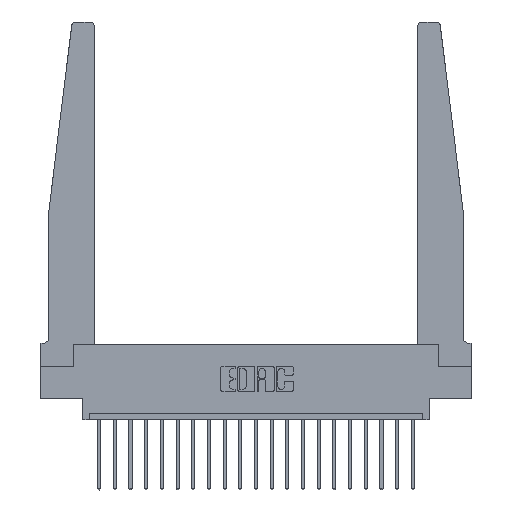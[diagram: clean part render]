
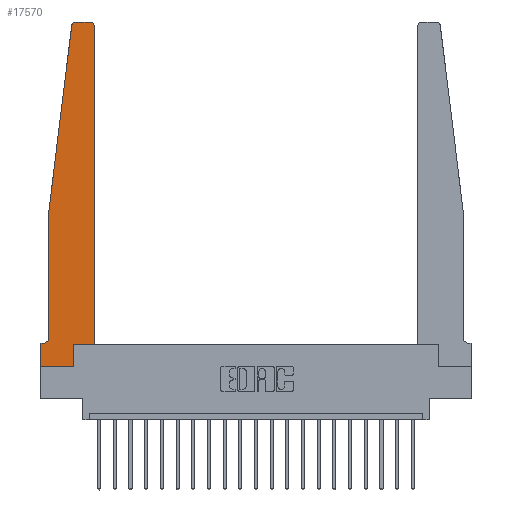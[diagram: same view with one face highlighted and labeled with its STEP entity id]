
A CAD part, top view. The second image highlights one B-rep face of the part: STEP entity #17570.
In plain terms, the highlighted planar face has unit normal (0, 0, 1).
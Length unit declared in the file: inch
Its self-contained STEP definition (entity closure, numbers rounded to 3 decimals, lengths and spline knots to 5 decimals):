
#269 = CARTESIAN_POINT ( 'NONE',  ( 0.395, 2.72, 0.37 ) ) ;
#278 = DIRECTION ( 'NONE',  ( 1., 0., 0. ) ) ;
#320 = LINE ( 'NONE', #11941, #8382 ) ;
#343 = ORIENTED_EDGE ( 'NONE', *, *, #20203, .T. ) ;
#544 = DIRECTION ( 'NONE',  ( 1., 0., 0. ) ) ;
#1042 = VERTEX_POINT ( 'NONE', #15136 ) ;
#1136 = VECTOR ( 'NONE', #544, 39.37008 ) ;
#1371 = VERTEX_POINT ( 'NONE', #17434 ) ;
#1635 = ORIENTED_EDGE ( 'NONE', *, *, #14695, .T. ) ;
#1880 = ORIENTED_EDGE ( 'NONE', *, *, #18486, .T. ) ;
#2098 = CARTESIAN_POINT ( 'NONE',  ( 0.2605, 0.18, 0.37 ) ) ;
#2448 = CARTESIAN_POINT ( 'NONE',  ( 0.015, 0.1875, 0.37 ) ) ;
#2742 = VECTOR ( 'NONE', #6853, 39.37008 ) ;
#2832 = DIRECTION ( 'NONE',  ( 0., -1., 0. ) ) ;
#3207 = EDGE_CURVE ( 'NONE', #11237, #1042, #18487, .T. ) ;
#3303 = DIRECTION ( 'NONE',  ( 0., 1., 0. ) ) ;
#3375 = CARTESIAN_POINT ( 'NONE',  ( 0.065, 1.25, 0.37 ) ) ;
#3447 = VECTOR ( 'NONE', #17825, 39.37008 ) ;
#3812 = ORIENTED_EDGE ( 'NONE', *, *, #11074, .T. ) ;
#3903 = DIRECTION ( 'NONE',  ( 1., 0., 0. ) ) ;
#4135 = EDGE_CURVE ( 'NONE', #15339, #16574, #13714, .T. ) ;
#4387 = VECTOR ( 'NONE', #2832, 39.37008 ) ;
#4436 = CARTESIAN_POINT ( 'NONE',  ( 0.015, 0.2375, 0.37 ) ) ;
#4474 = CARTESIAN_POINT ( 'NONE',  ( 0.27653, 2.75, 0.37 ) ) ;
#4518 = EDGE_CURVE ( 'NONE', #4698, #8866, #16947, .T. ) ;
#4573 = DIRECTION ( 'NONE',  ( -1., 0., 0. ) ) ;
#4656 = VECTOR ( 'NONE', #12025, 39.37008 ) ;
#4698 = VERTEX_POINT ( 'NONE', #2098 ) ;
#4708 = AXIS2_PLACEMENT_3D ( 'NONE', #16289, #14747, #278 ) ;
#4717 = DIRECTION ( 'NONE',  ( 0., 0., -1. ) ) ;
#4794 = DIRECTION ( 'NONE',  ( 0., 0., 1. ) ) ;
#4830 = CIRCLE ( 'NONE', #19026, 0.03 ) ;
#5326 = ORIENTED_EDGE ( 'NONE', *, *, #11999, .T. ) ;
#5350 = CARTESIAN_POINT ( 'NONE',  ( 0.425, 0.18, 0.37 ) ) ;
#6739 = ORIENTED_EDGE ( 'NONE', *, *, #17157, .T. ) ;
#6757 = CIRCLE ( 'NONE', #13583, 0.03 ) ;
#6811 = CARTESIAN_POINT ( 'NONE',  ( 0.27653, 2.72, 0.37 ) ) ;
#6853 = DIRECTION ( 'NONE',  ( -0.122, -0.992, 0. ) ) ;
#7519 = CARTESIAN_POINT ( 'NONE',  ( 0., 0.1875, 0.37 ) ) ;
#7604 = CARTESIAN_POINT ( 'NONE',  ( 0.065, 1.25, 0.37 ) ) ;
#7938 = EDGE_LOOP ( 'NONE', ( #10064, #1635, #12003, #343, #18929, #3812, #11332, #6739, #5326, #16904, #19817, #1880 ) ) ;
#7961 = VECTOR ( 'NONE', #3303, 39.37008 ) ;
#8055 = CARTESIAN_POINT ( 'NONE',  ( 0.24675, 2.72367, 0.37 ) ) ;
#8382 = VECTOR ( 'NONE', #15225, 39.37008 ) ;
#8735 = CARTESIAN_POINT ( 'NONE',  ( 0.25, 2.75, 0.37 ) ) ;
#8866 = VERTEX_POINT ( 'NONE', #13699 ) ;
#8931 = LINE ( 'NONE', #8735, #4656 ) ;
#9279 = EDGE_CURVE ( 'NONE', #8866, #1371, #11989, .T. ) ;
#9654 = LINE ( 'NONE', #10292, #11390 ) ;
#10027 = CARTESIAN_POINT ( 'NONE',  ( 0.065, 0.2375, 0.37 ) ) ;
#10064 = ORIENTED_EDGE ( 'NONE', *, *, #10383, .T. ) ;
#10292 = CARTESIAN_POINT ( 'NONE',  ( 0.2605, 0.18, 0.37 ) ) ;
#10306 = VECTOR ( 'NONE', #3903, 39.37008 ) ;
#10383 = EDGE_CURVE ( 'NONE', #11871, #17810, #8931, .T. ) ;
#10805 = VERTEX_POINT ( 'NONE', #3375 ) ;
#10965 = CARTESIAN_POINT ( 'NONE',  ( 0.2605, 0., 0.37 ) ) ;
#11074 = EDGE_CURVE ( 'NONE', #16574, #11237, #320, .T. ) ;
#11237 = VERTEX_POINT ( 'NONE', #7519 ) ;
#11332 = ORIENTED_EDGE ( 'NONE', *, *, #3207, .T. ) ;
#11390 = VECTOR ( 'NONE', #16640, 39.37008 ) ;
#11807 = CARTESIAN_POINT ( 'NONE',  ( 0.065, 1.25, 0.37 ) ) ;
#11833 = DIRECTION ( 'NONE',  ( 1., 0., 0. ) ) ;
#11871 = VERTEX_POINT ( 'NONE', #14827 ) ;
#11941 = CARTESIAN_POINT ( 'NONE',  ( 0.065, 0.1875, 0.37 ) ) ;
#11989 = LINE ( 'NONE', #19005, #7961 ) ;
#11999 = EDGE_CURVE ( 'NONE', #16138, #4698, #9654, .T. ) ;
#12003 = ORIENTED_EDGE ( 'NONE', *, *, #17707, .T. ) ;
#12025 = DIRECTION ( 'NONE',  ( -1., 0., 0. ) ) ;
#13284 = FACE_OUTER_BOUND ( 'NONE', #7938, .T. ) ;
#13366 = DIRECTION ( 'NONE',  ( 0., 0., 1. ) ) ;
#13578 = CARTESIAN_POINT ( 'NONE',  ( 0., 0., 0.37 ) ) ;
#13583 = AXIS2_PLACEMENT_3D ( 'NONE', #269, #4794, #14193 ) ;
#13699 = CARTESIAN_POINT ( 'NONE',  ( 0.425, 0.18, 0.37 ) ) ;
#13714 = CIRCLE ( 'NONE', #16889, 0.05 ) ;
#14193 = DIRECTION ( 'NONE',  ( 1., 0., 0. ) ) ;
#14493 = CARTESIAN_POINT ( 'NONE',  ( 0., 0., 0.37 ) ) ;
#14695 = EDGE_CURVE ( 'NONE', #17810, #15176, #4830, .T. ) ;
#14747 = DIRECTION ( 'NONE',  ( 0., 0., 1. ) ) ;
#14827 = CARTESIAN_POINT ( 'NONE',  ( 0.395, 2.75, 0.37 ) ) ;
#15136 = CARTESIAN_POINT ( 'NONE',  ( 0., 0., 0.37 ) ) ;
#15176 = VERTEX_POINT ( 'NONE', #8055 ) ;
#15225 = DIRECTION ( 'NONE',  ( -1., 0., 0. ) ) ;
#15339 = VERTEX_POINT ( 'NONE', #10027 ) ;
#16138 = VERTEX_POINT ( 'NONE', #10965 ) ;
#16289 = CARTESIAN_POINT ( 'NONE',  ( 0., 0.1875, 0.37 ) ) ;
#16574 = VERTEX_POINT ( 'NONE', #2448 ) ;
#16640 = DIRECTION ( 'NONE',  ( 0., 1., 0. ) ) ;
#16889 = AXIS2_PLACEMENT_3D ( 'NONE', #4436, #4717, #4573 ) ;
#16904 = ORIENTED_EDGE ( 'NONE', *, *, #4518, .T. ) ;
#16947 = LINE ( 'NONE', #5350, #1136 ) ;
#17157 = EDGE_CURVE ( 'NONE', #1042, #16138, #20547, .T. ) ;
#17434 = CARTESIAN_POINT ( 'NONE',  ( 0.425, 2.72, 0.37 ) ) ;
#17570 = ADVANCED_FACE ( 'NONE', ( #13284 ), #17739, .T. ) ;
#17707 = EDGE_CURVE ( 'NONE', #15176, #10805, #20017, .T. ) ;
#17739 = PLANE ( 'NONE',  #4708 ) ;
#17810 = VERTEX_POINT ( 'NONE', #4474 ) ;
#17825 = DIRECTION ( 'NONE',  ( 0., -1., 0. ) ) ;
#17915 = LINE ( 'NONE', #7604, #4387 ) ;
#18486 = EDGE_CURVE ( 'NONE', #1371, #11871, #6757, .T. ) ;
#18487 = LINE ( 'NONE', #14493, #3447 ) ;
#18929 = ORIENTED_EDGE ( 'NONE', *, *, #4135, .T. ) ;
#19005 = CARTESIAN_POINT ( 'NONE',  ( 0.425, 0.18, 0.37 ) ) ;
#19026 = AXIS2_PLACEMENT_3D ( 'NONE', #6811, #13366, #11833 ) ;
#19817 = ORIENTED_EDGE ( 'NONE', *, *, #9279, .T. ) ;
#20017 = LINE ( 'NONE', #11807, #2742 ) ;
#20203 = EDGE_CURVE ( 'NONE', #10805, #15339, #17915, .T. ) ;
#20547 = LINE ( 'NONE', #13578, #10306 ) ;
